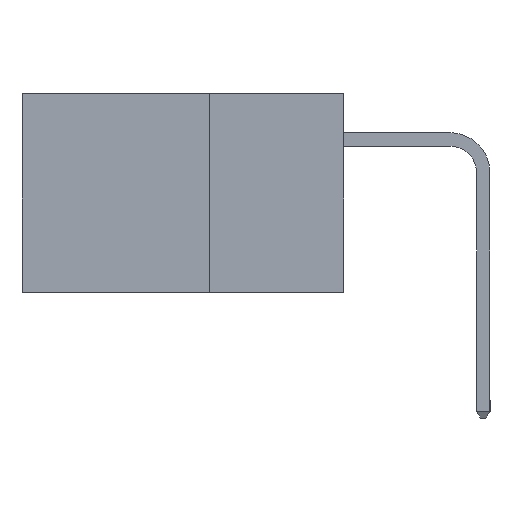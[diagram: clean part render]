
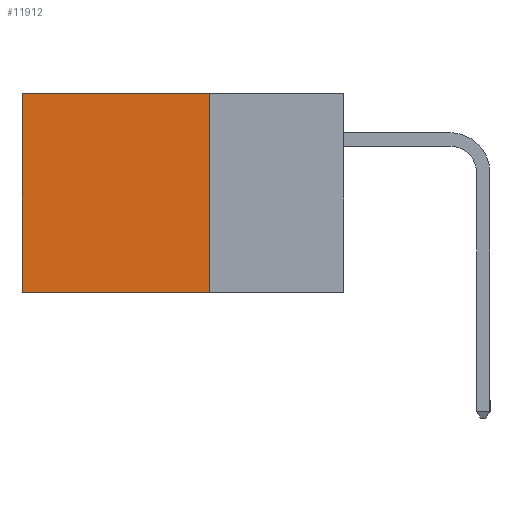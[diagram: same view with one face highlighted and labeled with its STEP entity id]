
A CAD part, left-side view. The second image highlights one B-rep face of the part: STEP entity #11912.
In plain terms, the highlighted planar face has unit normal (-1, 0, 0).
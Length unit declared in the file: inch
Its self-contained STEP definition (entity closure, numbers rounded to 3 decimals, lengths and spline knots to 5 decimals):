
#69 = ORIENTED_EDGE ( 'NONE', *, *, #12808, .F. ) ;
#468 = FACE_OUTER_BOUND ( 'NONE', #12995, .T. ) ;
#758 = ORIENTED_EDGE ( 'NONE', *, *, #13890, .F. ) ;
#1292 = VERTEX_POINT ( 'NONE', #1897 ) ;
#1601 = PLANE ( 'NONE',  #14729 ) ;
#1709 = DIRECTION ( 'NONE',  ( 1., 0., 0. ) ) ;
#1897 = CARTESIAN_POINT ( 'NONE',  ( 0.2615, 0.6, -0.37 ) ) ;
#3308 = LINE ( 'NONE', #8271, #12578 ) ;
#3533 = DIRECTION ( 'NONE',  ( 0., 0., -1. ) ) ;
#4147 = LINE ( 'NONE', #11208, #10095 ) ;
#4238 = ORIENTED_EDGE ( 'NONE', *, *, #13466, .T. ) ;
#4343 = VECTOR ( 'NONE', #15098, 39.37008 ) ;
#5078 = CARTESIAN_POINT ( 'NONE',  ( 0.2615, 0.25, -0.37 ) ) ;
#5300 = LINE ( 'NONE', #5361, #8106 ) ;
#5361 = CARTESIAN_POINT ( 'NONE',  ( 0.2615, 0.25, -0.37 ) ) ;
#5407 = VERTEX_POINT ( 'NONE', #11942 ) ;
#6114 = VERTEX_POINT ( 'NONE', #5078 ) ;
#6700 = CARTESIAN_POINT ( 'NONE',  ( 0.2615, 0.25, 0. ) ) ;
#6777 = LINE ( 'NONE', #6700, #4343 ) ;
#7547 = ORIENTED_EDGE ( 'NONE', *, *, #7939, .T. ) ;
#7688 = VERTEX_POINT ( 'NONE', #8316 ) ;
#7762 = CARTESIAN_POINT ( 'NONE',  ( 0.2615, 0.25, -0.37 ) ) ;
#7939 = EDGE_CURVE ( 'NONE', #7688, #1292, #3308, .T. ) ;
#8106 = VECTOR ( 'NONE', #13705, 39.37008 ) ;
#8271 = CARTESIAN_POINT ( 'NONE',  ( 0.2615, 0.6, -0.37 ) ) ;
#8316 = CARTESIAN_POINT ( 'NONE',  ( 0.2615, 0.6, 0. ) ) ;
#10095 = VECTOR ( 'NONE', #12390, 39.37008 ) ;
#11208 = CARTESIAN_POINT ( 'NONE',  ( 0.2615, 0.25, -0.37 ) ) ;
#11912 = ADVANCED_FACE ( 'NONE', ( #468 ), #1601, .F. ) ;
#11942 = CARTESIAN_POINT ( 'NONE',  ( 0.2615, 0.25, 0. ) ) ;
#12390 = DIRECTION ( 'NONE',  ( 0., 1., 0. ) ) ;
#12410 = DIRECTION ( 'NONE',  ( 0., 0., -1. ) ) ;
#12578 = VECTOR ( 'NONE', #3533, 39.37008 ) ;
#12808 = EDGE_CURVE ( 'NONE', #5407, #6114, #5300, .T. ) ;
#12995 = EDGE_LOOP ( 'NONE', ( #7547, #758, #69, #4238 ) ) ;
#13466 = EDGE_CURVE ( 'NONE', #5407, #7688, #6777, .T. ) ;
#13705 = DIRECTION ( 'NONE',  ( 0., 0., -1. ) ) ;
#13890 = EDGE_CURVE ( 'NONE', #6114, #1292, #4147, .T. ) ;
#14729 = AXIS2_PLACEMENT_3D ( 'NONE', #7762, #1709, #12410 ) ;
#15098 = DIRECTION ( 'NONE',  ( 0., 1., 0. ) ) ;
